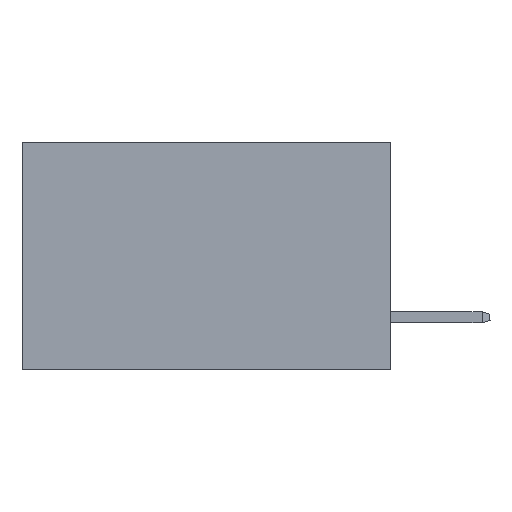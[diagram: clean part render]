
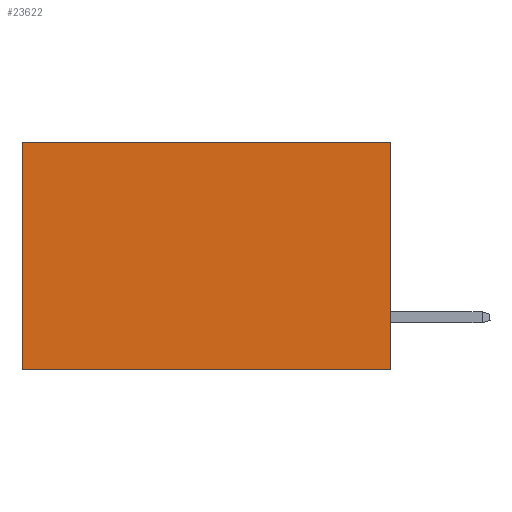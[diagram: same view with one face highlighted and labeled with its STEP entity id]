
A CAD part, left-side view. The second image highlights one B-rep face of the part: STEP entity #23622.
In plain terms, the highlighted planar face has unit normal (-1, 0, 0).
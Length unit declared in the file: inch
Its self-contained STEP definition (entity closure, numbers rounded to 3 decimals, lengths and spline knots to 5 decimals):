
#256 = DIRECTION ( 'NONE',  ( 0., 0., -1. ) ) ;
#404 = CARTESIAN_POINT ( 'NONE',  ( 0.2875, 0., 0. ) ) ;
#2178 = ORIENTED_EDGE ( 'NONE', *, *, #17044, .F. ) ;
#2489 = CARTESIAN_POINT ( 'NONE',  ( 0.2875, 0., 0. ) ) ;
#2811 = DIRECTION ( 'NONE',  ( 0., 1., 0. ) ) ;
#3082 = FACE_OUTER_BOUND ( 'NONE', #4793, .T. ) ;
#3382 = DIRECTION ( 'NONE',  ( 0., 0., -1. ) ) ;
#4793 = EDGE_LOOP ( 'NONE', ( #21094, #22416, #2178, #8010 ) ) ;
#5623 = VERTEX_POINT ( 'NONE', #21540 ) ;
#5803 = EDGE_CURVE ( 'NONE', #21708, #15486, #15264, .T. ) ;
#6886 = CARTESIAN_POINT ( 'NONE',  ( 0.2875, 0.6, 0. ) ) ;
#7362 = PLANE ( 'NONE',  #22821 ) ;
#8010 = ORIENTED_EDGE ( 'NONE', *, *, #22996, .T. ) ;
#9050 = VECTOR ( 'NONE', #2811, 39.37008 ) ;
#12986 = VECTOR ( 'NONE', #3382, 39.37008 ) ;
#14377 = DIRECTION ( 'NONE',  ( 1., 0., 0. ) ) ;
#14496 = LINE ( 'NONE', #404, #9050 ) ;
#14552 = VECTOR ( 'NONE', #29229, 39.37008 ) ;
#15264 = LINE ( 'NONE', #26917, #14552 ) ;
#15486 = VERTEX_POINT ( 'NONE', #23612 ) ;
#16266 = CARTESIAN_POINT ( 'NONE',  ( 0.2875, 0., -0.37 ) ) ;
#17044 = EDGE_CURVE ( 'NONE', #18092, #21708, #18307, .T. ) ;
#18092 = VERTEX_POINT ( 'NONE', #2489 ) ;
#18307 = LINE ( 'NONE', #24331, #12986 ) ;
#20207 = LINE ( 'NONE', #6886, #26398 ) ;
#21094 = ORIENTED_EDGE ( 'NONE', *, *, #22794, .T. ) ;
#21540 = CARTESIAN_POINT ( 'NONE',  ( 0.2875, 0.6, 0. ) ) ;
#21708 = VERTEX_POINT ( 'NONE', #16266 ) ;
#22416 = ORIENTED_EDGE ( 'NONE', *, *, #5803, .F. ) ;
#22794 = EDGE_CURVE ( 'NONE', #5623, #15486, #20207, .T. ) ;
#22821 = AXIS2_PLACEMENT_3D ( 'NONE', #28164, #14377, #256 ) ;
#22996 = EDGE_CURVE ( 'NONE', #18092, #5623, #14496, .T. ) ;
#23051 = DIRECTION ( 'NONE',  ( 0., 0., -1. ) ) ;
#23612 = CARTESIAN_POINT ( 'NONE',  ( 0.2875, 0.6, -0.37 ) ) ;
#23622 = ADVANCED_FACE ( 'NONE', ( #3082 ), #7362, .F. ) ;
#24331 = CARTESIAN_POINT ( 'NONE',  ( 0.2875, 0., 0. ) ) ;
#26398 = VECTOR ( 'NONE', #23051, 39.37008 ) ;
#26917 = CARTESIAN_POINT ( 'NONE',  ( 0.2875, 0., -0.37 ) ) ;
#28164 = CARTESIAN_POINT ( 'NONE',  ( 0.2875, 0., 0. ) ) ;
#29229 = DIRECTION ( 'NONE',  ( 0., 1., 0. ) ) ;
